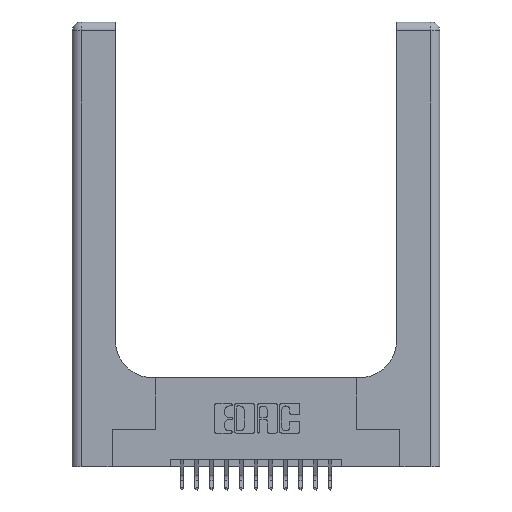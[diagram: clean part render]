
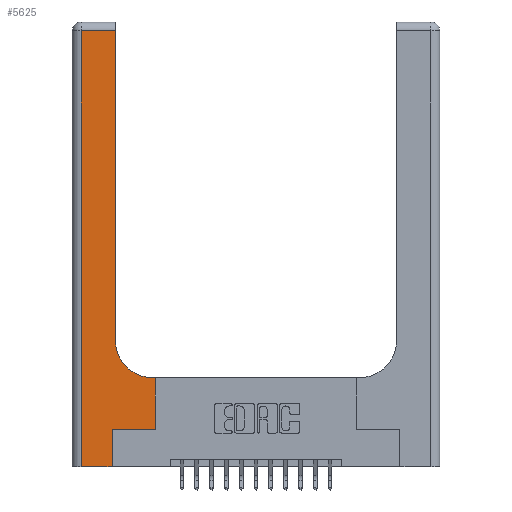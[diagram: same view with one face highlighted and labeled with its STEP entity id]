
A CAD part, top view. The second image highlights one B-rep face of the part: STEP entity #5625.
In plain terms, the highlighted planar face has unit normal (0, 0, 1).
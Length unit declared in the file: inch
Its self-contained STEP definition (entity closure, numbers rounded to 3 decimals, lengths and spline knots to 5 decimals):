
#133 = CARTESIAN_POINT ( 'NONE',  ( 0.269, 0., 0.37 ) ) ;
#140 = ORIENTED_EDGE ( 'NONE', *, *, #17006, .T. ) ;
#383 = CARTESIAN_POINT ( 'NONE',  ( 0.5415, 0.6, 0.37 ) ) ;
#950 = LINE ( 'NONE', #9114, #16799 ) ;
#1068 = CARTESIAN_POINT ( 'NONE',  ( 0.2915, 0.85, 0.37 ) ) ;
#1121 = CARTESIAN_POINT ( 'NONE',  ( 0.5585, 0.6, 0.37 ) ) ;
#1649 = LINE ( 'NONE', #11031, #17492 ) ;
#1684 = EDGE_CURVE ( 'NONE', #6028, #7845, #7718, .T. ) ;
#1868 = DIRECTION ( 'NONE',  ( -1., 0., 0. ) ) ;
#2225 = CARTESIAN_POINT ( 'NONE',  ( 0.06, 3., 0.37 ) ) ;
#2238 = VECTOR ( 'NONE', #1868, 39.37008 ) ;
#2581 = DIRECTION ( 'NONE',  ( 1., 0., 0. ) ) ;
#2979 = CARTESIAN_POINT ( 'NONE',  ( 0.5585, 0.25, 0.37 ) ) ;
#3281 = VERTEX_POINT ( 'NONE', #133 ) ;
#3729 = ORIENTED_EDGE ( 'NONE', *, *, #8589, .T. ) ;
#3778 = DIRECTION ( 'NONE',  ( 0., 1., 0. ) ) ;
#4067 = DIRECTION ( 'NONE',  ( 0., 0., -1. ) ) ;
#4293 = CARTESIAN_POINT ( 'NONE',  ( 0.5585, 0.25, 0.37 ) ) ;
#4326 = CARTESIAN_POINT ( 'NONE',  ( 0.2915, 3., 0.37 ) ) ;
#4357 = DIRECTION ( 'NONE',  ( 0., 0., -1. ) ) ;
#4486 = VERTEX_POINT ( 'NONE', #14054 ) ;
#4598 = CARTESIAN_POINT ( 'NONE',  ( 0., 3., 0.37 ) ) ;
#4777 = VECTOR ( 'NONE', #5582, 39.37008 ) ;
#4815 = CARTESIAN_POINT ( 'NONE',  ( 0.06, 0., 0.37 ) ) ;
#5410 = AXIS2_PLACEMENT_3D ( 'NONE', #4598, #4357, #5771 ) ;
#5516 = ORIENTED_EDGE ( 'NONE', *, *, #9994, .T. ) ;
#5582 = DIRECTION ( 'NONE',  ( 0., 1., 0. ) ) ;
#5625 = ADVANCED_FACE ( 'NONE', ( #10415 ), #15836, .F. ) ;
#5771 = DIRECTION ( 'NONE',  ( -1., 0., 0. ) ) ;
#5940 = CARTESIAN_POINT ( 'NONE',  ( 0.2915, 2.94, 0.37 ) ) ;
#5947 = EDGE_CURVE ( 'NONE', #3281, #16694, #12154, .T. ) ;
#6028 = VERTEX_POINT ( 'NONE', #1068 ) ;
#6613 = AXIS2_PLACEMENT_3D ( 'NONE', #12444, #4067, #15293 ) ;
#6618 = CIRCLE ( 'NONE', #6613, 0.25 ) ;
#6769 = EDGE_CURVE ( 'NONE', #13386, #3281, #1649, .T. ) ;
#7718 = LINE ( 'NONE', #4326, #16749 ) ;
#7788 = ORIENTED_EDGE ( 'NONE', *, *, #11013, .T. ) ;
#7845 = VERTEX_POINT ( 'NONE', #5940 ) ;
#7997 = VECTOR ( 'NONE', #3778, 39.37008 ) ;
#8589 = EDGE_CURVE ( 'NONE', #10033, #11877, #16323, .T. ) ;
#8857 = ORIENTED_EDGE ( 'NONE', *, *, #10144, .T. ) ;
#8921 = DIRECTION ( 'NONE',  ( -1., 0., 0. ) ) ;
#9114 = CARTESIAN_POINT ( 'NONE',  ( 0.269, 0.25, 0.37 ) ) ;
#9331 = CARTESIAN_POINT ( 'NONE',  ( 0.269, 0., 0.37 ) ) ;
#9994 = EDGE_CURVE ( 'NONE', #4486, #13386, #11413, .T. ) ;
#10033 = VERTEX_POINT ( 'NONE', #1121 ) ;
#10144 = EDGE_CURVE ( 'NONE', #11877, #6028, #6618, .T. ) ;
#10415 = FACE_OUTER_BOUND ( 'NONE', #10606, .T. ) ;
#10484 = VECTOR ( 'NONE', #8921, 39.37008 ) ;
#10606 = EDGE_LOOP ( 'NONE', ( #11885, #7788, #5516, #14171, #14764, #140, #17854, #3729, #8857 ) ) ;
#11013 = EDGE_CURVE ( 'NONE', #7845, #4486, #12915, .T. ) ;
#11031 = CARTESIAN_POINT ( 'NONE',  ( 0., 0., 0.37 ) ) ;
#11413 = LINE ( 'NONE', #2225, #12737 ) ;
#11531 = DIRECTION ( 'NONE',  ( 0., 1., 0. ) ) ;
#11877 = VERTEX_POINT ( 'NONE', #383 ) ;
#11885 = ORIENTED_EDGE ( 'NONE', *, *, #1684, .T. ) ;
#12154 = LINE ( 'NONE', #9331, #7997 ) ;
#12444 = CARTESIAN_POINT ( 'NONE',  ( 0.5415, 0.85, 0.37 ) ) ;
#12459 = EDGE_CURVE ( 'NONE', #17458, #10033, #14847, .T. ) ;
#12737 = VECTOR ( 'NONE', #16375, 39.37008 ) ;
#12915 = LINE ( 'NONE', #17382, #10484 ) ;
#13386 = VERTEX_POINT ( 'NONE', #4815 ) ;
#14054 = CARTESIAN_POINT ( 'NONE',  ( 0.06, 2.94, 0.37 ) ) ;
#14171 = ORIENTED_EDGE ( 'NONE', *, *, #6769, .T. ) ;
#14764 = ORIENTED_EDGE ( 'NONE', *, *, #5947, .T. ) ;
#14847 = LINE ( 'NONE', #2979, #4777 ) ;
#15187 = CARTESIAN_POINT ( 'NONE',  ( 0.2915, 0.6, 0.37 ) ) ;
#15293 = DIRECTION ( 'NONE',  ( 1., 0., 0. ) ) ;
#15836 = PLANE ( 'NONE',  #5410 ) ;
#16217 = DIRECTION ( 'NONE',  ( 1., 0., 0. ) ) ;
#16323 = LINE ( 'NONE', #15187, #2238 ) ;
#16375 = DIRECTION ( 'NONE',  ( 0., -1., 0. ) ) ;
#16694 = VERTEX_POINT ( 'NONE', #16961 ) ;
#16749 = VECTOR ( 'NONE', #11531, 39.37008 ) ;
#16799 = VECTOR ( 'NONE', #16217, 39.37008 ) ;
#16961 = CARTESIAN_POINT ( 'NONE',  ( 0.269, 0.25, 0.37 ) ) ;
#17006 = EDGE_CURVE ( 'NONE', #16694, #17458, #950, .T. ) ;
#17382 = CARTESIAN_POINT ( 'NONE',  ( 0., 2.94, 0.37 ) ) ;
#17458 = VERTEX_POINT ( 'NONE', #4293 ) ;
#17492 = VECTOR ( 'NONE', #2581, 39.37008 ) ;
#17854 = ORIENTED_EDGE ( 'NONE', *, *, #12459, .T. ) ;
